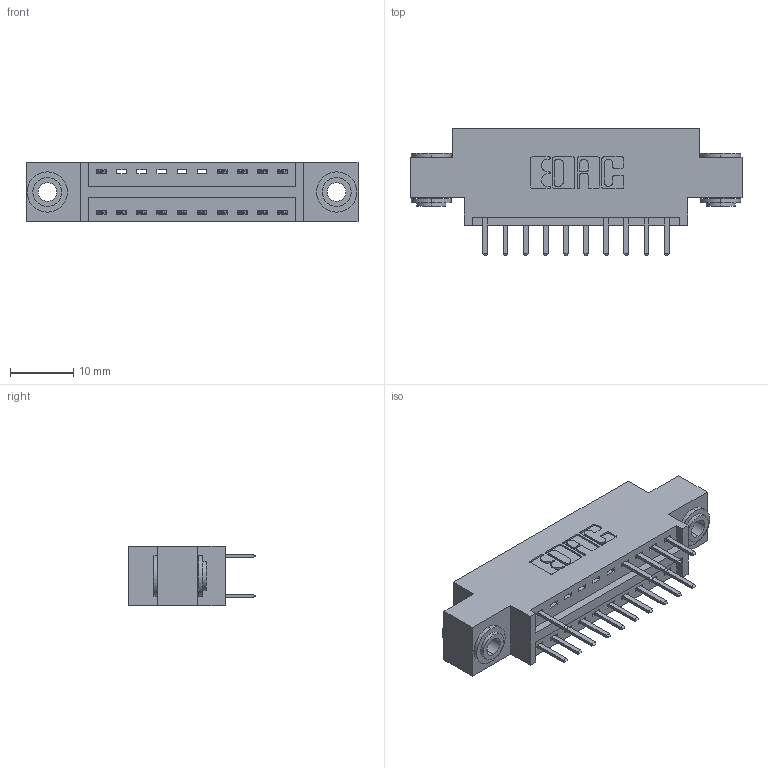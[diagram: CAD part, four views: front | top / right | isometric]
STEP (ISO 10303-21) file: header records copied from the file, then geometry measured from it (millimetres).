
FILE_DESCRIPTION (( 'STEP AP203' ), '1' );
FILE_NAME ('346-020-520-803.STEP', '2018-08-20T11:11:22', ( '' ), ( '' ), 'SwSTEP 2.0', 'SolidWorks 2016', '' );
FILE_SCHEMA (( 'CONFIG_CONTROL_DESIGN' ));
Length unit declared in the file: inch
Products named in the file (4): 345-292-001_345-293-120; 345-250-002_345-250-002-102; 346-020-520-803; 346 Part_0.170 Offset - 0.156 Dia-TH
Assembly tree (18 placements, depth 2):
  346-020-520-803
    346 Part_0.170 Offset - 0.156 Dia-TH
    345-292-001_345-293-120  x15
    345-250-002_345-250-002-102  x2
Bounding box: 52.32 x 20.02 x 9.4 mm (x, y, z)
Volume: 4666.9 mm3; surface area: 6030.9 mm2
Topology: 18 solids, 18 shells, 1034 faces, 2967 edges, 1934 vertices
Faces by surface type: plane 670, cylinder 356, cone 8
Entity records: 11570 total; most frequent: CARTESIAN_POINT 1962, ORIENTED_EDGE 1882, DIRECTION 1793, EDGE_CURVE 941, LINE 741, VECTOR 741, VERTEX_POINT 622, AXIS2_PLACEMENT_3D 526
